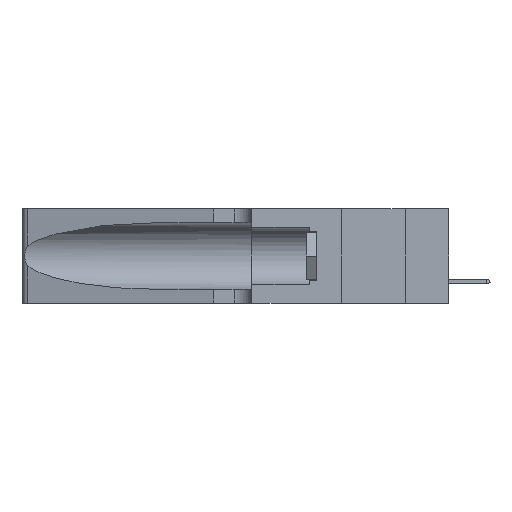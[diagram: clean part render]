
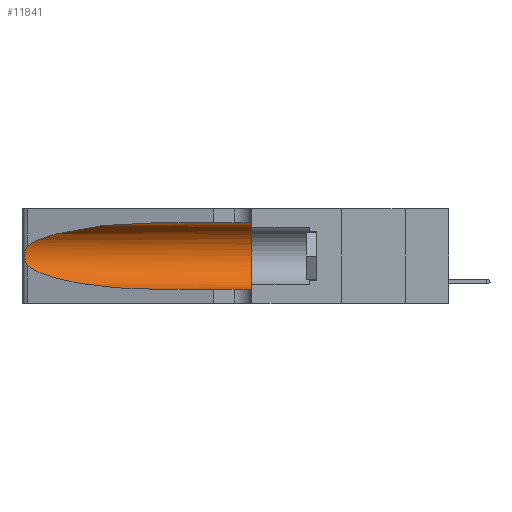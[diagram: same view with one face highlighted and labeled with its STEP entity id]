
A CAD part, left-side view. The second image highlights one B-rep face of the part: STEP entity #11841.
In plain terms, the highlighted cylindrical face has radius 3.308 mm (diameter 6.617 mm), a partial arc.
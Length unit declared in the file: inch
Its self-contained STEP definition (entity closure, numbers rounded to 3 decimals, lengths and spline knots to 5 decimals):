
#274 = CARTESIAN_POINT ( 'NONE',  ( 0.18966, 0.96281, 0.05475 ) ) ;
#1177 = DIRECTION ( 'NONE',  ( 0., -1., 0. ) ) ;
#1391 = VERTEX_POINT ( 'NONE', #4129 ) ;
#1899 = CARTESIAN_POINT ( 'NONE',  ( 0.25555, 1.22993, 0.14849 ) ) ;
#2099 = EDGE_CURVE ( 'NONE', #15367, #1391, #7980, .T. ) ;
#2263 = CARTESIAN_POINT ( 'NONE',  ( 0.2373, 1.15595, 0.08982 ) ) ;
#3097 =( BOUNDED_CURVE ( )  B_SPLINE_CURVE ( 3, ( #3294, #4060, #20688, #26802 ),
 .UNSPECIFIED., .F., .F. ) 
 B_SPLINE_CURVE_WITH_KNOTS ( ( 4, 4 ),
 ( 1.5708, 2.84003 ),
 .UNSPECIFIED. ) 
 CURVE ( )  GEOMETRIC_REPRESENTATION_ITEM ( )  RATIONAL_B_SPLINE_CURVE ( ( 1., 0.87, 0.87, 1. ) ) 
 REPRESENTATION_ITEM ( '' )  );
#3294 = CARTESIAN_POINT ( 'NONE',  ( 0.1305, 0.72297, 0.31525 ) ) ;
#3596 = VERTEX_POINT ( 'NONE', #6711 ) ;
#4060 = CARTESIAN_POINT ( 'NONE',  ( 0.18966, 0.96281, 0.31525 ) ) ;
#4129 = CARTESIAN_POINT ( 'NONE',  ( 0.1305, 0.35, 0.31525 ) ) ;
#4885 = CARTESIAN_POINT ( 'NONE',  ( 0.1305, 0.35, 0.185 ) ) ;
#4953 = EDGE_CURVE ( 'NONE', #21970, #3596, #23726, .T. ) ;
#6010 = CARTESIAN_POINT ( 'NONE',  ( 0.25787, 1.23484, 0.2124 ) ) ;
#6209 = ORIENTED_EDGE ( 'NONE', *, *, #2099, .F. ) ;
#6711 = CARTESIAN_POINT ( 'NONE',  ( 0.25487, 1.22718, 0.14631 ) ) ;
#6932 = DIRECTION ( 'NONE',  ( 0., 1., 0. ) ) ;
#6963 = FACE_OUTER_BOUND ( 'NONE', #22733, .T. ) ;
#7980 = LINE ( 'NONE', #11456, #12188 ) ;
#10087 = DIRECTION ( 'NONE',  ( 0., -1., 0. ) ) ;
#10127 = CARTESIAN_POINT ( 'NONE',  ( 0.25487, 1.22718, 0.14631 ) ) ;
#10231 = CARTESIAN_POINT ( 'NONE',  ( 0.25789, 1.23486, 0.15765 ) ) ;
#10316 = CARTESIAN_POINT ( 'NONE',  ( 0.25856, 1.23593, 0.16098 ) ) ;
#10411 = CARTESIAN_POINT ( 'NONE',  ( 0.26075, 1.23896, 0.178 ) ) ;
#10497 = CARTESIAN_POINT ( 'NONE',  ( 0.1305, 1.61858, 0.05475 ) ) ;
#10755 = DIRECTION ( 'NONE',  ( 0., -1., 0. ) ) ;
#11239 = CARTESIAN_POINT ( 'NONE',  ( 0.1305, 0.72297, 0.05475 ) ) ;
#11456 = CARTESIAN_POINT ( 'NONE',  ( 0.1305, 1.61858, 0.31525 ) ) ;
#11841 = ADVANCED_FACE ( 'NONE', ( #6963 ), #21037, .F. ) ;
#12188 = VECTOR ( 'NONE', #1177, 39.37008 ) ;
#12236 = CARTESIAN_POINT ( 'NONE',  ( 0.25555, 1.22994, 0.2215 ) ) ;
#12415 = CARTESIAN_POINT ( 'NONE',  ( 0.25639, 1.23186, 0.15144 ) ) ;
#12946 = CARTESIAN_POINT ( 'NONE',  ( 0.1305, 0.35, 0.05475 ) ) ;
#14446 = CARTESIAN_POINT ( 'NONE',  ( 0.25487, 1.22718, 0.22369 ) ) ;
#14455 = ORIENTED_EDGE ( 'NONE', *, *, #15546, .F. ) ;
#15367 = VERTEX_POINT ( 'NONE', #26945 ) ;
#15546 = EDGE_CURVE ( 'NONE', #1391, #20138, #20649, .T. ) ;
#15710 = ORIENTED_EDGE ( 'NONE', *, *, #19038, .T. ) ;
#16228 = VERTEX_POINT ( 'NONE', #20491 ) ;
#16490 = CARTESIAN_POINT ( 'NONE',  ( 0.26018, 1.23835, 0.19895 ) ) ;
#16548 =( BOUNDED_CURVE ( )  B_SPLINE_CURVE ( 3, ( #16838, #2263, #274, #11239 ),
 .UNSPECIFIED., .F., .F. ) 
 B_SPLINE_CURVE_WITH_KNOTS ( ( 4, 4 ),
 ( 3.44316, 4.71239 ),
 .UNSPECIFIED. ) 
 CURVE ( )  GEOMETRIC_REPRESENTATION_ITEM ( )  RATIONAL_B_SPLINE_CURVE ( ( 1., 0.87, 0.87, 1. ) ) 
 REPRESENTATION_ITEM ( '' )  );
#16838 = CARTESIAN_POINT ( 'NONE',  ( 0.25487, 1.22718, 0.14631 ) ) ;
#17122 = ORIENTED_EDGE ( 'NONE', *, *, #17522, .T. ) ;
#17522 = EDGE_CURVE ( 'NONE', #15367, #21970, #3097, .T. ) ;
#18803 = DIRECTION ( 'NONE',  ( 0., 0., -1. ) ) ;
#19038 = EDGE_CURVE ( 'NONE', #16228, #20138, #20480, .T. ) ;
#20138 = VERTEX_POINT ( 'NONE', #12946 ) ;
#20305 = AXIS2_PLACEMENT_3D ( 'NONE', #4885, #6932, #25693 ) ;
#20314 = CARTESIAN_POINT ( 'NONE',  ( 0.1305, 1.61858, 0.185 ) ) ;
#20480 = LINE ( 'NONE', #10497, #21090 ) ;
#20491 = CARTESIAN_POINT ( 'NONE',  ( 0.1305, 0.72297, 0.05475 ) ) ;
#20649 = CIRCLE ( 'NONE', #20305, 0.13025 ) ;
#20683 = CARTESIAN_POINT ( 'NONE',  ( 0.26075, 1.23896, 0.19203 ) ) ;
#20688 = CARTESIAN_POINT ( 'NONE',  ( 0.2373, 1.15595, 0.28018 ) ) ;
#20862 = CARTESIAN_POINT ( 'NONE',  ( 0.26017, 1.23833, 0.17102 ) ) ;
#21037 = CYLINDRICAL_SURFACE ( 'NONE', #22694, 0.13025 ) ;
#21090 = VECTOR ( 'NONE', #10755, 39.37008 ) ;
#21970 = VERTEX_POINT ( 'NONE', #24927 ) ;
#22630 = EDGE_CURVE ( 'NONE', #3596, #16228, #16548, .T. ) ;
#22694 = AXIS2_PLACEMENT_3D ( 'NONE', #20314, #10087, #18803 ) ;
#22733 = EDGE_LOOP ( 'NONE', ( #17122, #26068, #25380, #15710, #14455, #6209 ) ) ;
#23726 = B_SPLINE_CURVE_WITH_KNOTS ( 'NONE', 3,
 ( #14446, #12236, #24978, #6010, #26987, #16490, #20683, #10411, #20862, #10316, #10231, #12415, #1899, #10127 ),
 .UNSPECIFIED., .F., .F.,
 ( 4, 2, 2, 2, 2, 2, 4 ),
 ( 0., 0.00027, 0.00053, 0.00107, 0.0016, 0.00187, 0.00214 ),
 .UNSPECIFIED. ) ;
#24927 = CARTESIAN_POINT ( 'NONE',  ( 0.25487, 1.22718, 0.22369 ) ) ;
#24978 = CARTESIAN_POINT ( 'NONE',  ( 0.25639, 1.23184, 0.21858 ) ) ;
#25380 = ORIENTED_EDGE ( 'NONE', *, *, #22630, .T. ) ;
#25693 = DIRECTION ( 'NONE',  ( 0., 0., 1. ) ) ;
#26068 = ORIENTED_EDGE ( 'NONE', *, *, #4953, .T. ) ;
#26802 = CARTESIAN_POINT ( 'NONE',  ( 0.25487, 1.22718, 0.22369 ) ) ;
#26945 = CARTESIAN_POINT ( 'NONE',  ( 0.1305, 0.72297, 0.31525 ) ) ;
#26987 = CARTESIAN_POINT ( 'NONE',  ( 0.25854, 1.2359, 0.20912 ) ) ;
